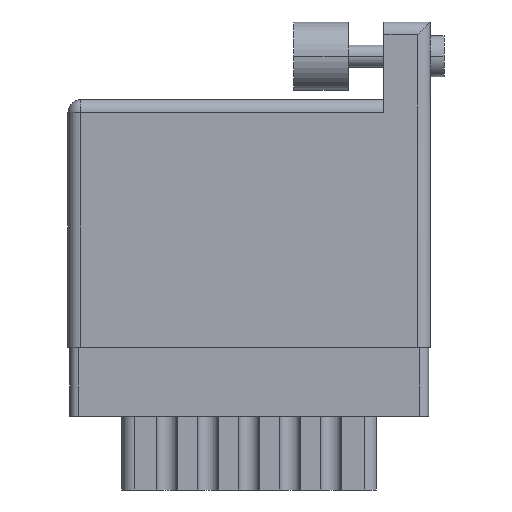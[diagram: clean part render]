
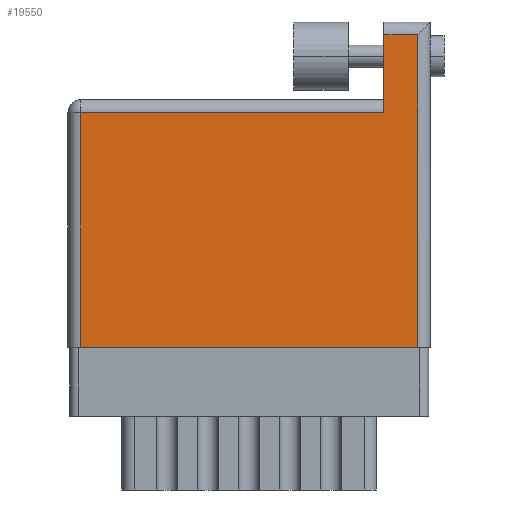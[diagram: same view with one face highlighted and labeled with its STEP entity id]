
A CAD part, front view. The second image highlights one B-rep face of the part: STEP entity #19550.
In plain terms, the highlighted face is planar.
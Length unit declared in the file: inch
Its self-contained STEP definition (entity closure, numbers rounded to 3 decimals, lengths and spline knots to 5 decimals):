
#33 = CARTESIAN_POINT ( 'NONE',  ( 1.155, 1.143, 0. ) ) ;
#95 = DIRECTION ( 'NONE',  ( 1., 0., 0. ) ) ;
#767 = ORIENTED_EDGE ( 'NONE', *, *, #22741, .T. ) ;
#941 = CARTESIAN_POINT ( 'NONE',  ( 1.155, 1.143, 0. ) ) ;
#2021 = EDGE_CURVE ( 'NONE', #23481, #23062, #4104, .T. ) ;
#2298 = CARTESIAN_POINT ( 'NONE',  ( 0., 0., 0. ) ) ;
#2746 = VERTEX_POINT ( 'NONE', #6819 ) ;
#3094 = VERTEX_POINT ( 'NONE', #14607 ) ;
#3233 = EDGE_CURVE ( 'NONE', #3094, #2746, #16282, .T. ) ;
#4024 = VECTOR ( 'NONE', #16236, 39.37008 ) ;
#4104 = LINE ( 'NONE', #6048, #19476 ) ;
#4207 = DIRECTION ( 'NONE',  ( -1., 0., 0. ) ) ;
#4462 = ORIENTED_EDGE ( 'NONE', *, *, #2021, .T. ) ;
#4534 = EDGE_LOOP ( 'NONE', ( #19318, #21763, #23691, #4462, #767, #18380 ) ) ;
#4651 = AXIS2_PLACEMENT_3D ( 'NONE', #23416, #5331, #21605 ) ;
#5331 = DIRECTION ( 'NONE',  ( 0., 0., -1. ) ) ;
#6048 = CARTESIAN_POINT ( 'NONE',  ( 1.155, 1.19, 0. ) ) ;
#6311 = LINE ( 'NONE', #14250, #11266 ) ;
#6557 = VERTEX_POINT ( 'NONE', #19415 ) ;
#6819 = CARTESIAN_POINT ( 'NONE',  ( 1.278, 1.143, 0. ) ) ;
#8927 = CARTESIAN_POINT ( 'NONE',  ( 0.047, 0., 0. ) ) ;
#9937 = LINE ( 'NONE', #33, #10472 ) ;
#10171 = CARTESIAN_POINT ( 'NONE',  ( 1.278, 1.19, 0. ) ) ;
#10472 = VECTOR ( 'NONE', #4207, 39.37008 ) ;
#11266 = VECTOR ( 'NONE', #12294, 39.37008 ) ;
#12172 = VERTEX_POINT ( 'NONE', #8927 ) ;
#12294 = DIRECTION ( 'NONE',  ( 0., -1., 0. ) ) ;
#12322 = CARTESIAN_POINT ( 'NONE',  ( 0., 0.859, 0. ) ) ;
#12739 = VECTOR ( 'NONE', #95, 39.37008 ) ;
#14197 = DIRECTION ( 'NONE',  ( 0., 1., 0. ) ) ;
#14250 = CARTESIAN_POINT ( 'NONE',  ( 0.047, 0., 0. ) ) ;
#14508 = VECTOR ( 'NONE', #14197, 39.37008 ) ;
#14607 = CARTESIAN_POINT ( 'NONE',  ( 1.278, 0., 0. ) ) ;
#16236 = DIRECTION ( 'NONE',  ( -1., 0., 0. ) ) ;
#16282 = LINE ( 'NONE', #10171, #14508 ) ;
#17250 = CARTESIAN_POINT ( 'NONE',  ( 1.155, 0.859, 0. ) ) ;
#17303 = FACE_OUTER_BOUND ( 'NONE', #4534, .T. ) ;
#18380 = ORIENTED_EDGE ( 'NONE', *, *, #18726, .T. ) ;
#18726 = EDGE_CURVE ( 'NONE', #6557, #12172, #6311, .T. ) ;
#19005 = EDGE_CURVE ( 'NONE', #2746, #23481, #9937, .T. ) ;
#19318 = ORIENTED_EDGE ( 'NONE', *, *, #22761, .T. ) ;
#19415 = CARTESIAN_POINT ( 'NONE',  ( 0.047, 0.859, 0. ) ) ;
#19476 = VECTOR ( 'NONE', #24133, 39.37008 ) ;
#19550 = ADVANCED_FACE ( 'NONE', ( #17303 ), #19767, .F. ) ;
#19767 = PLANE ( 'NONE',  #4651 ) ;
#20514 = LINE ( 'NONE', #12322, #4024 ) ;
#21605 = DIRECTION ( 'NONE',  ( -1., 0., 0. ) ) ;
#21763 = ORIENTED_EDGE ( 'NONE', *, *, #3233, .T. ) ;
#22333 = LINE ( 'NONE', #2298, #12739 ) ;
#22741 = EDGE_CURVE ( 'NONE', #23062, #6557, #20514, .T. ) ;
#22761 = EDGE_CURVE ( 'NONE', #12172, #3094, #22333, .T. ) ;
#23062 = VERTEX_POINT ( 'NONE', #17250 ) ;
#23416 = CARTESIAN_POINT ( 'NONE',  ( 0., 0.906, 0. ) ) ;
#23481 = VERTEX_POINT ( 'NONE', #941 ) ;
#23691 = ORIENTED_EDGE ( 'NONE', *, *, #19005, .T. ) ;
#24133 = DIRECTION ( 'NONE',  ( 0., -1., 0. ) ) ;
